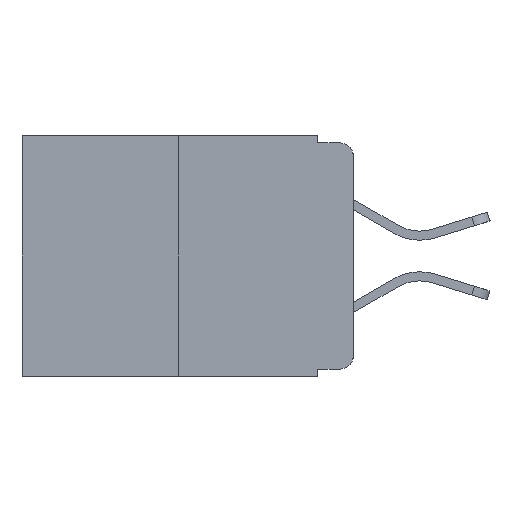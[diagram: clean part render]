
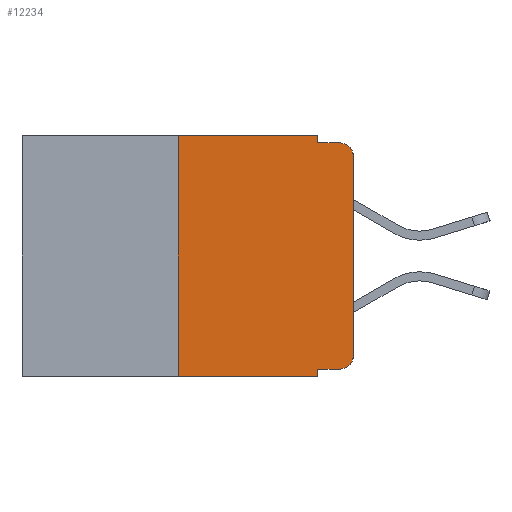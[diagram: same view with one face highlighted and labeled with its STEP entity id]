
A CAD part, left-side view. The second image highlights one B-rep face of the part: STEP entity #12234.
In plain terms, the highlighted planar face has unit normal (-1, 0, 0).
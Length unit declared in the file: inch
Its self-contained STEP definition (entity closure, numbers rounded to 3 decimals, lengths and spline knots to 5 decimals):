
#24 = VERTEX_POINT ( 'NONE', #19467 ) ;
#99 = ORIENTED_EDGE ( 'NONE', *, *, #17579, .F. ) ;
#200 = ORIENTED_EDGE ( 'NONE', *, *, #11893, .T. ) ;
#376 = VECTOR ( 'NONE', #14735, 39.37008 ) ;
#388 = DIRECTION ( 'NONE',  ( 0., -1., 0. ) ) ;
#399 = ORIENTED_EDGE ( 'NONE', *, *, #23550, .F. ) ;
#810 = DIRECTION ( 'NONE',  ( 0., 0., 1. ) ) ;
#1649 = LINE ( 'NONE', #11003, #20567 ) ;
#1832 = VERTEX_POINT ( 'NONE', #13663 ) ;
#2272 = EDGE_CURVE ( 'NONE', #7773, #5848, #7288, .T. ) ;
#2564 = DIRECTION ( 'NONE',  ( 0., 0., -1. ) ) ;
#2741 = CARTESIAN_POINT ( 'NONE',  ( 0., 0.25, 0. ) ) ;
#3154 = VECTOR ( 'NONE', #810, 39.37008 ) ;
#3431 = VECTOR ( 'NONE', #388, 39.37008 ) ;
#3680 = DIRECTION ( 'NONE',  ( 0., 0., 1. ) ) ;
#4080 = LINE ( 'NONE', #5134, #8944 ) ;
#4824 = ORIENTED_EDGE ( 'NONE', *, *, #2272, .T. ) ;
#5134 = CARTESIAN_POINT ( 'NONE',  ( 0., 0.051, 0. ) ) ;
#5703 = CARTESIAN_POINT ( 'NONE',  ( 0., 0., -0.313 ) ) ;
#5848 = VERTEX_POINT ( 'NONE', #19356 ) ;
#6130 = VERTEX_POINT ( 'NONE', #16458 ) ;
#6215 = VERTEX_POINT ( 'NONE', #5703 ) ;
#6575 = ORIENTED_EDGE ( 'NONE', *, *, #7834, .T. ) ;
#6790 = CARTESIAN_POINT ( 'NONE',  ( 0., 0.02, -0.03 ) ) ;
#7224 = ORIENTED_EDGE ( 'NONE', *, *, #23107, .F. ) ;
#7236 = AXIS2_PLACEMENT_3D ( 'NONE', #6790, #19541, #8607 ) ;
#7288 = LINE ( 'NONE', #18456, #19552 ) ;
#7458 = LINE ( 'NONE', #15435, #17222 ) ;
#7677 = CIRCLE ( 'NONE', #7236, 0.02 ) ;
#7750 = LINE ( 'NONE', #13363, #3431 ) ;
#7773 = VERTEX_POINT ( 'NONE', #8337 ) ;
#7834 = EDGE_CURVE ( 'NONE', #1832, #6215, #22624, .T. ) ;
#8231 = CARTESIAN_POINT ( 'NONE',  ( 0., 0.051, -0.01 ) ) ;
#8337 = CARTESIAN_POINT ( 'NONE',  ( 0., 0.25, -0.343 ) ) ;
#8494 = CARTESIAN_POINT ( 'NONE',  ( 0., 0.02, -0.313 ) ) ;
#8607 = DIRECTION ( 'NONE',  ( 0., 0., -1. ) ) ;
#8944 = VECTOR ( 'NONE', #19755, 39.37008 ) ;
#9557 = DIRECTION ( 'NONE',  ( 1., 0., 0. ) ) ;
#10328 = DIRECTION ( 'NONE',  ( 0., 0., -1. ) ) ;
#10502 = FACE_OUTER_BOUND ( 'NONE', #15821, .T. ) ;
#10543 = EDGE_CURVE ( 'NONE', #6215, #13844, #1649, .T. ) ;
#11003 = CARTESIAN_POINT ( 'NONE',  ( 0., 0., 0. ) ) ;
#11124 = CARTESIAN_POINT ( 'NONE',  ( 0., 0., -0.03 ) ) ;
#11355 = VECTOR ( 'NONE', #11959, 39.37008 ) ;
#11513 = EDGE_CURVE ( 'NONE', #19581, #1832, #15162, .T. ) ;
#11766 = ORIENTED_EDGE ( 'NONE', *, *, #10543, .T. ) ;
#11893 = EDGE_CURVE ( 'NONE', #13844, #24, #7677, .T. ) ;
#11958 = VERTEX_POINT ( 'NONE', #23218 ) ;
#11959 = DIRECTION ( 'NONE',  ( 0., -1., 0. ) ) ;
#12234 = ADVANCED_FACE ( 'NONE', ( #10502 ), #20470, .F. ) ;
#12334 = CARTESIAN_POINT ( 'NONE',  ( 0., 0.25, 0. ) ) ;
#12489 = LINE ( 'NONE', #8231, #11355 ) ;
#12577 = ORIENTED_EDGE ( 'NONE', *, *, #12805, .F. ) ;
#12805 = EDGE_CURVE ( 'NONE', #6130, #24, #12489, .T. ) ;
#12891 = CARTESIAN_POINT ( 'NONE',  ( 0., 0.051, -0.333 ) ) ;
#12968 = ORIENTED_EDGE ( 'NONE', *, *, #11513, .T. ) ;
#13363 = CARTESIAN_POINT ( 'NONE',  ( 0., 0.473, 0. ) ) ;
#13663 = CARTESIAN_POINT ( 'NONE',  ( 0., 0.02, -0.333 ) ) ;
#13844 = VERTEX_POINT ( 'NONE', #11124 ) ;
#14068 = LINE ( 'NONE', #2741, #3154 ) ;
#14644 = ORIENTED_EDGE ( 'NONE', *, *, #16156, .F. ) ;
#14735 = DIRECTION ( 'NONE',  ( 0., -1., 0. ) ) ;
#14864 = DIRECTION ( 'NONE',  ( 0., -1., 0. ) ) ;
#15034 = CARTESIAN_POINT ( 'NONE',  ( 0., 0.473, 0. ) ) ;
#15162 = LINE ( 'NONE', #12891, #376 ) ;
#15398 = AXIS2_PLACEMENT_3D ( 'NONE', #15034, #9557, #22232 ) ;
#15435 = CARTESIAN_POINT ( 'NONE',  ( 0., 0.051, 0. ) ) ;
#15821 = EDGE_LOOP ( 'NONE', ( #11766, #200, #12577, #14644, #99, #7224, #4824, #399, #12968, #6575 ) ) ;
#16156 = EDGE_CURVE ( 'NONE', #11958, #6130, #4080, .T. ) ;
#16458 = CARTESIAN_POINT ( 'NONE',  ( 0., 0.051, -0.01 ) ) ;
#17222 = VECTOR ( 'NONE', #2564, 39.37008 ) ;
#17327 = AXIS2_PLACEMENT_3D ( 'NONE', #8494, #21200, #10328 ) ;
#17579 = EDGE_CURVE ( 'NONE', #18474, #11958, #7750, .T. ) ;
#18456 = CARTESIAN_POINT ( 'NONE',  ( 0., 0.473, -0.343 ) ) ;
#18474 = VERTEX_POINT ( 'NONE', #12334 ) ;
#19356 = CARTESIAN_POINT ( 'NONE',  ( 0., 0.051, -0.343 ) ) ;
#19467 = CARTESIAN_POINT ( 'NONE',  ( 0., 0.02, -0.01 ) ) ;
#19541 = DIRECTION ( 'NONE',  ( -1., 0., 0. ) ) ;
#19552 = VECTOR ( 'NONE', #14864, 39.37008 ) ;
#19581 = VERTEX_POINT ( 'NONE', #21231 ) ;
#19755 = DIRECTION ( 'NONE',  ( 0., 0., -1. ) ) ;
#20470 = PLANE ( 'NONE',  #15398 ) ;
#20567 = VECTOR ( 'NONE', #3680, 39.37008 ) ;
#21200 = DIRECTION ( 'NONE',  ( -1., 0., 0. ) ) ;
#21231 = CARTESIAN_POINT ( 'NONE',  ( 0., 0.051, -0.333 ) ) ;
#22232 = DIRECTION ( 'NONE',  ( 0., 0., -1. ) ) ;
#22624 = CIRCLE ( 'NONE', #17327, 0.02 ) ;
#23107 = EDGE_CURVE ( 'NONE', #7773, #18474, #14068, .T. ) ;
#23218 = CARTESIAN_POINT ( 'NONE',  ( 0., 0.051, 0. ) ) ;
#23550 = EDGE_CURVE ( 'NONE', #19581, #5848, #7458, .T. ) ;
